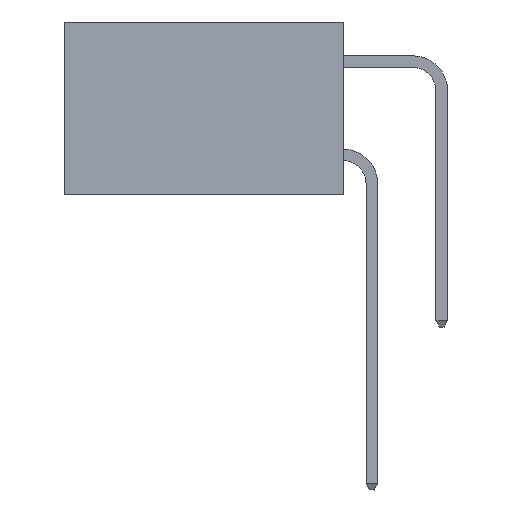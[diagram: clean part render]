
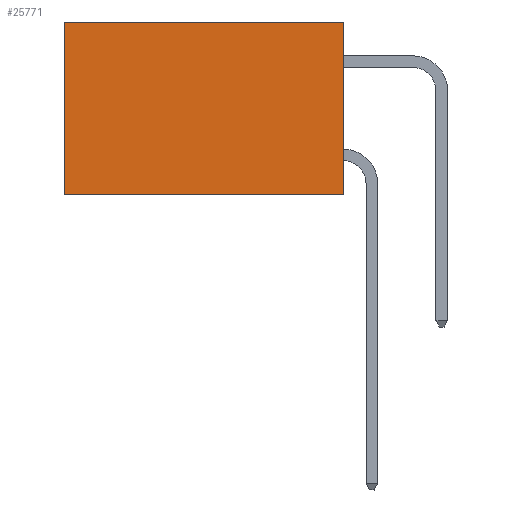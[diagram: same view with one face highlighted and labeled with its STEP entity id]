
A CAD part, left-side view. The second image highlights one B-rep face of the part: STEP entity #25771.
In plain terms, the highlighted planar face has unit normal (-1, 0, 0).
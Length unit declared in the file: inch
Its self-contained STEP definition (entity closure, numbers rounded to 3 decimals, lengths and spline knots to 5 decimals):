
#1674 = CARTESIAN_POINT ( 'NONE',  ( 0.298, 0., -0.37 ) ) ;
#1879 = EDGE_CURVE ( 'NONE', #5014, #9628, #20489, .T. ) ;
#5014 = VERTEX_POINT ( 'NONE', #11453 ) ;
#7376 = VECTOR ( 'NONE', #23617, 39.37008 ) ;
#7973 = CARTESIAN_POINT ( 'NONE',  ( 0.298, 0., -0.37 ) ) ;
#9628 = VERTEX_POINT ( 'NONE', #7973 ) ;
#10218 = EDGE_CURVE ( 'NONE', #5014, #24526, #14382, .T. ) ;
#11236 = CARTESIAN_POINT ( 'NONE',  ( 0.298, 0., 0. ) ) ;
#11453 = CARTESIAN_POINT ( 'NONE',  ( 0.298, 0., 0. ) ) ;
#12043 = VECTOR ( 'NONE', #32602, 39.37008 ) ;
#12279 = CARTESIAN_POINT ( 'NONE',  ( 0.298, 0.6, 0. ) ) ;
#12847 = LINE ( 'NONE', #1674, #12043 ) ;
#12910 = CARTESIAN_POINT ( 'NONE',  ( 0.298, 0.6, -0.37 ) ) ;
#13504 = CARTESIAN_POINT ( 'NONE',  ( 0.298, 0., 0. ) ) ;
#13559 = VECTOR ( 'NONE', #16114, 39.37008 ) ;
#13848 = DIRECTION ( 'NONE',  ( 0., 0., -1. ) ) ;
#14372 = ORIENTED_EDGE ( 'NONE', *, *, #1879, .F. ) ;
#14382 = LINE ( 'NONE', #13504, #13559 ) ;
#14910 = EDGE_CURVE ( 'NONE', #9628, #23405, #12847, .T. ) ;
#15370 = CARTESIAN_POINT ( 'NONE',  ( 0.298, 0.6, 0. ) ) ;
#15581 = ORIENTED_EDGE ( 'NONE', *, *, #14910, .F. ) ;
#15618 = EDGE_CURVE ( 'NONE', #24526, #23405, #31749, .T. ) ;
#16114 = DIRECTION ( 'NONE',  ( 0., 1., 0. ) ) ;
#18023 = DIRECTION ( 'NONE',  ( 0., 0., -1. ) ) ;
#18380 = VECTOR ( 'NONE', #18023, 39.37008 ) ;
#20094 = ORIENTED_EDGE ( 'NONE', *, *, #15618, .T. ) ;
#20489 = LINE ( 'NONE', #23683, #7376 ) ;
#22104 = ORIENTED_EDGE ( 'NONE', *, *, #10218, .T. ) ;
#22617 = FACE_OUTER_BOUND ( 'NONE', #25134, .T. ) ;
#23405 = VERTEX_POINT ( 'NONE', #12910 ) ;
#23617 = DIRECTION ( 'NONE',  ( 0., 0., -1. ) ) ;
#23683 = CARTESIAN_POINT ( 'NONE',  ( 0.298, 0., 0. ) ) ;
#24296 = AXIS2_PLACEMENT_3D ( 'NONE', #11236, #29083, #13848 ) ;
#24526 = VERTEX_POINT ( 'NONE', #12279 ) ;
#25134 = EDGE_LOOP ( 'NONE', ( #20094, #15581, #14372, #22104 ) ) ;
#25771 = ADVANCED_FACE ( 'NONE', ( #22617 ), #26608, .F. ) ;
#26608 = PLANE ( 'NONE',  #24296 ) ;
#29083 = DIRECTION ( 'NONE',  ( 1., 0., 0. ) ) ;
#31749 = LINE ( 'NONE', #15370, #18380 ) ;
#32602 = DIRECTION ( 'NONE',  ( 0., 1., 0. ) ) ;
